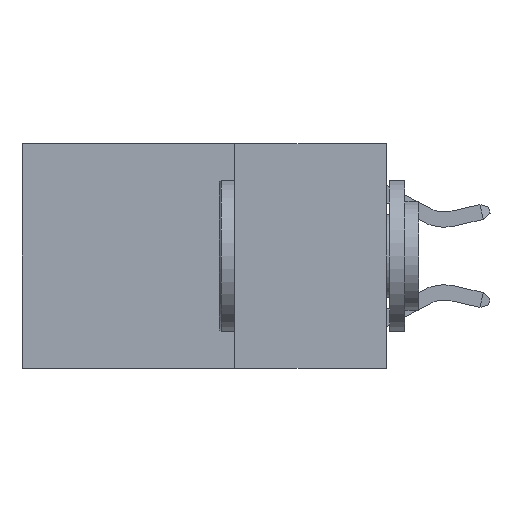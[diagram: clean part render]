
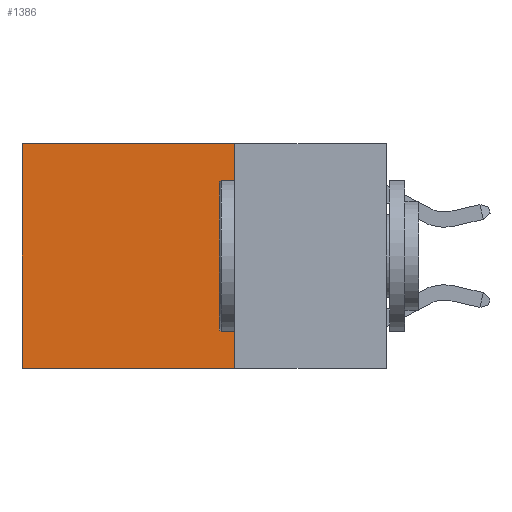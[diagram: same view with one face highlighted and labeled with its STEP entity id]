
A CAD part, left-side view. The second image highlights one B-rep face of the part: STEP entity #1386.
In plain terms, the highlighted planar face has unit normal (-1, 0, 0).
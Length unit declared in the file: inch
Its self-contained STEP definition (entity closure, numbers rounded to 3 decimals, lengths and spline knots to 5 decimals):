
#928 = FACE_OUTER_BOUND ( 'NONE', #3233, .T. ) ;
#1044 = PLANE ( 'NONE',  #4312 ) ;
#1136 = DIRECTION ( 'NONE',  ( 0., 0., -1. ) ) ;
#1386 = ADVANCED_FACE ( 'NONE', ( #928 ), #1044, .F. ) ;
#1399 = EDGE_CURVE ( 'NONE', #12224, #7964, #2320, .T. ) ;
#1458 = VERTEX_POINT ( 'NONE', #11054 ) ;
#2129 = VECTOR ( 'NONE', #13978, 39.37008 ) ;
#2320 = LINE ( 'NONE', #5355, #6082 ) ;
#3198 = DIRECTION ( 'NONE',  ( 0., 1., 0. ) ) ;
#3233 = EDGE_LOOP ( 'NONE', ( #12289, #6665, #7134, #7984 ) ) ;
#3361 = VECTOR ( 'NONE', #7310, 39.37008 ) ;
#3489 = CARTESIAN_POINT ( 'NONE',  ( 0.2625, 0.6, 0. ) ) ;
#4312 = AXIS2_PLACEMENT_3D ( 'NONE', #6422, #14230, #1136 ) ;
#4905 = CARTESIAN_POINT ( 'NONE',  ( 0.2625, 0.25, 0. ) ) ;
#5031 = CARTESIAN_POINT ( 'NONE',  ( 0.2625, 0.25, 0. ) ) ;
#5355 = CARTESIAN_POINT ( 'NONE',  ( 0.2625, 0.25, 0. ) ) ;
#6082 = VECTOR ( 'NONE', #12097, 39.37008 ) ;
#6173 = CARTESIAN_POINT ( 'NONE',  ( 0.2625, 0.6, 0. ) ) ;
#6422 = CARTESIAN_POINT ( 'NONE',  ( 0.2625, 0.25, 0. ) ) ;
#6450 = CARTESIAN_POINT ( 'NONE',  ( 0.2625, 0.25, -0.37 ) ) ;
#6538 = VECTOR ( 'NONE', #3198, 39.37008 ) ;
#6665 = ORIENTED_EDGE ( 'NONE', *, *, #8765, .F. ) ;
#7134 = ORIENTED_EDGE ( 'NONE', *, *, #12868, .F. ) ;
#7144 = EDGE_CURVE ( 'NONE', #7964, #1458, #7788, .T. ) ;
#7310 = DIRECTION ( 'NONE',  ( 0., 0., -1. ) ) ;
#7788 = LINE ( 'NONE', #6173, #2129 ) ;
#7964 = VERTEX_POINT ( 'NONE', #3489 ) ;
#7984 = ORIENTED_EDGE ( 'NONE', *, *, #1399, .T. ) ;
#8765 = EDGE_CURVE ( 'NONE', #9582, #1458, #13463, .T. ) ;
#9582 = VERTEX_POINT ( 'NONE', #9591 ) ;
#9591 = CARTESIAN_POINT ( 'NONE',  ( 0.2625, 0.25, -0.37 ) ) ;
#11054 = CARTESIAN_POINT ( 'NONE',  ( 0.2625, 0.6, -0.37 ) ) ;
#12097 = DIRECTION ( 'NONE',  ( 0., 1., 0. ) ) ;
#12224 = VERTEX_POINT ( 'NONE', #4905 ) ;
#12289 = ORIENTED_EDGE ( 'NONE', *, *, #7144, .T. ) ;
#12336 = LINE ( 'NONE', #5031, #3361 ) ;
#12868 = EDGE_CURVE ( 'NONE', #12224, #9582, #12336, .T. ) ;
#13463 = LINE ( 'NONE', #6450, #6538 ) ;
#13978 = DIRECTION ( 'NONE',  ( 0., 0., -1. ) ) ;
#14230 = DIRECTION ( 'NONE',  ( 1., 0., 0. ) ) ;
